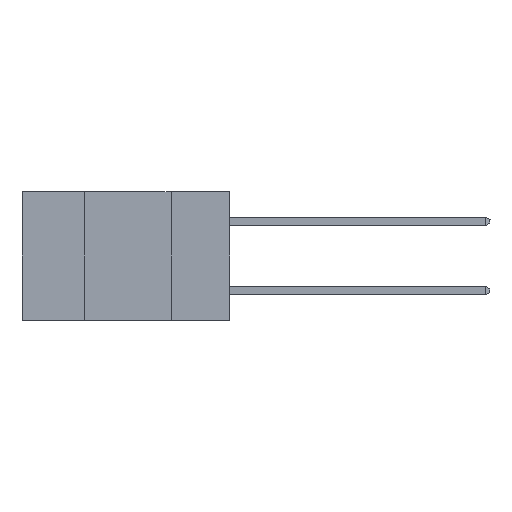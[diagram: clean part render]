
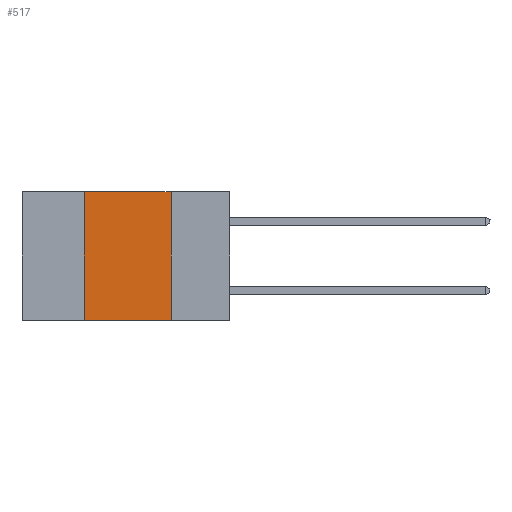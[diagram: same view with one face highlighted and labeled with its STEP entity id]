
A CAD part, left-side view. The second image highlights one B-rep face of the part: STEP entity #517.
In plain terms, the highlighted planar face has unit normal (-1, 0, 0).
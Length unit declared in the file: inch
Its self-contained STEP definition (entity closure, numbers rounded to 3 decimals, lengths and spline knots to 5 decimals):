
#15 = CARTESIAN_POINT ( 'NONE',  ( 0., 0.6, -0.37 ) ) ;
#517 = ADVANCED_FACE ( 'NONE', ( #6468 ), #24576, .F. ) ;
#1206 = CARTESIAN_POINT ( 'NONE',  ( 0., 0.42, -0.37 ) ) ;
#1877 = CARTESIAN_POINT ( 'NONE',  ( 0., 0.17, 0. ) ) ;
#2141 = VECTOR ( 'NONE', #11906, 39.37008 ) ;
#2212 = VECTOR ( 'NONE', #23782, 39.37008 ) ;
#2364 = VERTEX_POINT ( 'NONE', #24936 ) ;
#2755 = ORIENTED_EDGE ( 'NONE', *, *, #10819, .F. ) ;
#2988 = DIRECTION ( 'NONE',  ( 1., 0., 0. ) ) ;
#3001 = ORIENTED_EDGE ( 'NONE', *, *, #16370, .F. ) ;
#3326 = VERTEX_POINT ( 'NONE', #17130 ) ;
#3708 = EDGE_CURVE ( 'NONE', #22332, #2364, #18656, .T. ) ;
#4924 = ORIENTED_EDGE ( 'NONE', *, *, #3708, .F. ) ;
#5872 = DIRECTION ( 'NONE',  ( 0., 0., -1. ) ) ;
#6024 = EDGE_LOOP ( 'NONE', ( #2755, #4924, #3001, #13403 ) ) ;
#6468 = FACE_OUTER_BOUND ( 'NONE', #6024, .T. ) ;
#7052 = LINE ( 'NONE', #21659, #17532 ) ;
#7866 = DIRECTION ( 'NONE',  ( 0., 0., 1. ) ) ;
#9509 = EDGE_CURVE ( 'NONE', #13746, #3326, #23317, .T. ) ;
#10073 = CARTESIAN_POINT ( 'NONE',  ( 0., 0.6, 0. ) ) ;
#10819 = EDGE_CURVE ( 'NONE', #2364, #3326, #23258, .T. ) ;
#11906 = DIRECTION ( 'NONE',  ( 0., 0., -1. ) ) ;
#12812 = VECTOR ( 'NONE', #21037, 39.37008 ) ;
#13403 = ORIENTED_EDGE ( 'NONE', *, *, #9509, .T. ) ;
#13746 = VERTEX_POINT ( 'NONE', #1206 ) ;
#14453 = AXIS2_PLACEMENT_3D ( 'NONE', #10073, #2988, #5872 ) ;
#16370 = EDGE_CURVE ( 'NONE', #13746, #22332, #7052, .T. ) ;
#17086 = CARTESIAN_POINT ( 'NONE',  ( 0., 0.42, 0. ) ) ;
#17130 = CARTESIAN_POINT ( 'NONE',  ( 0., 0.17, -0.37 ) ) ;
#17532 = VECTOR ( 'NONE', #7866, 39.37008 ) ;
#18656 = LINE ( 'NONE', #20782, #12812 ) ;
#20782 = CARTESIAN_POINT ( 'NONE',  ( 0., 0.6, 0. ) ) ;
#21037 = DIRECTION ( 'NONE',  ( 0., -1., 0. ) ) ;
#21659 = CARTESIAN_POINT ( 'NONE',  ( 0., 0.42, 0. ) ) ;
#22332 = VERTEX_POINT ( 'NONE', #17086 ) ;
#23258 = LINE ( 'NONE', #1877, #2141 ) ;
#23317 = LINE ( 'NONE', #15, #2212 ) ;
#23782 = DIRECTION ( 'NONE',  ( 0., -1., 0. ) ) ;
#24576 = PLANE ( 'NONE',  #14453 ) ;
#24936 = CARTESIAN_POINT ( 'NONE',  ( 0., 0.17, 0. ) ) ;
